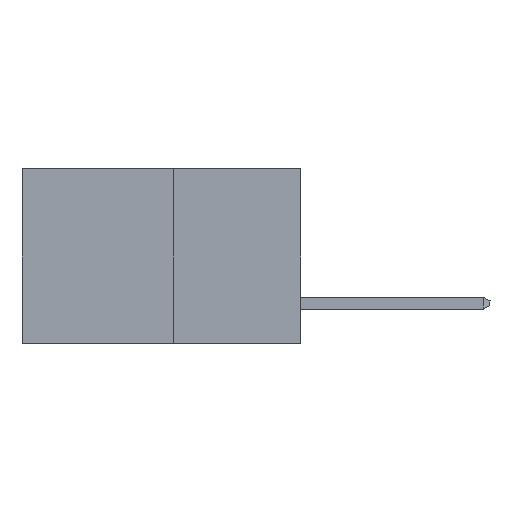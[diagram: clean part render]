
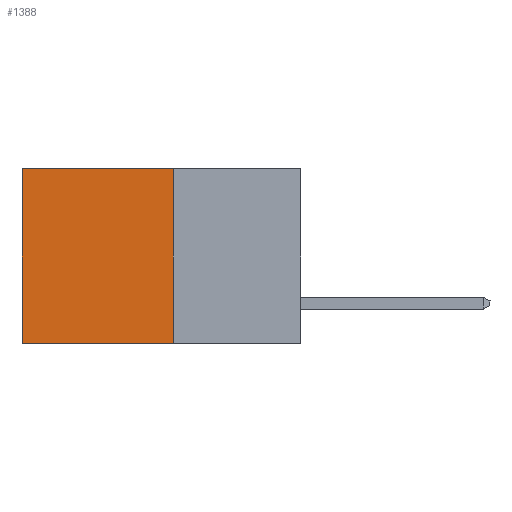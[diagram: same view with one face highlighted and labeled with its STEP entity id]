
A CAD part, left-side view. The second image highlights one B-rep face of the part: STEP entity #1388.
In plain terms, the highlighted planar face has unit normal (-1, 0, 0).
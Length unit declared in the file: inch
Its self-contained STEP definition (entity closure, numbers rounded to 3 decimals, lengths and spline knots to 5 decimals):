
#104 = LINE ( 'NONE', #6132, #11775 ) ;
#206 = DIRECTION ( 'NONE',  ( 0., 1., 0. ) ) ;
#1388 = ADVANCED_FACE ( 'NONE', ( #6121 ), #12274, .F. ) ;
#1566 = VERTEX_POINT ( 'NONE', #7856 ) ;
#3310 = EDGE_CURVE ( 'NONE', #8061, #10368, #8718, .T. ) ;
#3577 = CARTESIAN_POINT ( 'NONE',  ( 0.277, 0.59, -0.37 ) ) ;
#4282 = CARTESIAN_POINT ( 'NONE',  ( 0.277, 0.27, -0.37 ) ) ;
#4301 = DIRECTION ( 'NONE',  ( 1., 0., 0. ) ) ;
#5453 = EDGE_CURVE ( 'NONE', #8061, #1566, #104, .T. ) ;
#5772 = ORIENTED_EDGE ( 'NONE', *, *, #9436, .T. ) ;
#6121 = FACE_OUTER_BOUND ( 'NONE', #8485, .T. ) ;
#6132 = CARTESIAN_POINT ( 'NONE',  ( 0.277, 0.27, -0.37 ) ) ;
#6487 = ORIENTED_EDGE ( 'NONE', *, *, #9704, .F. ) ;
#7052 = VERTEX_POINT ( 'NONE', #3577 ) ;
#7252 = DIRECTION ( 'NONE',  ( 0., 0., -1. ) ) ;
#7275 = VECTOR ( 'NONE', #12536, 39.37008 ) ;
#7623 = ORIENTED_EDGE ( 'NONE', *, *, #5453, .F. ) ;
#7856 = CARTESIAN_POINT ( 'NONE',  ( 0.277, 0.27, -0.37 ) ) ;
#8061 = VERTEX_POINT ( 'NONE', #10741 ) ;
#8485 = EDGE_LOOP ( 'NONE', ( #5772, #6487, #7623, #8941 ) ) ;
#8579 = CARTESIAN_POINT ( 'NONE',  ( 0.277, 0.27, -0.37 ) ) ;
#8718 = LINE ( 'NONE', #11518, #14174 ) ;
#8941 = ORIENTED_EDGE ( 'NONE', *, *, #3310, .T. ) ;
#9164 = CARTESIAN_POINT ( 'NONE',  ( 0.277, 0.59, -0.37 ) ) ;
#9361 = LINE ( 'NONE', #4282, #12310 ) ;
#9436 = EDGE_CURVE ( 'NONE', #10368, #7052, #10226, .T. ) ;
#9578 = AXIS2_PLACEMENT_3D ( 'NONE', #8579, #4301, #10836 ) ;
#9704 = EDGE_CURVE ( 'NONE', #1566, #7052, #9361, .T. ) ;
#9876 = DIRECTION ( 'NONE',  ( 0., 1., 0. ) ) ;
#10226 = LINE ( 'NONE', #9164, #7275 ) ;
#10368 = VERTEX_POINT ( 'NONE', #14340 ) ;
#10741 = CARTESIAN_POINT ( 'NONE',  ( 0.277, 0.27, 0. ) ) ;
#10836 = DIRECTION ( 'NONE',  ( 0., 0., -1. ) ) ;
#11518 = CARTESIAN_POINT ( 'NONE',  ( 0.277, 0.27, 0. ) ) ;
#11775 = VECTOR ( 'NONE', #7252, 39.37008 ) ;
#12274 = PLANE ( 'NONE',  #9578 ) ;
#12310 = VECTOR ( 'NONE', #9876, 39.37008 ) ;
#12536 = DIRECTION ( 'NONE',  ( 0., 0., -1. ) ) ;
#14174 = VECTOR ( 'NONE', #206, 39.37008 ) ;
#14340 = CARTESIAN_POINT ( 'NONE',  ( 0.277, 0.59, 0. ) ) ;
